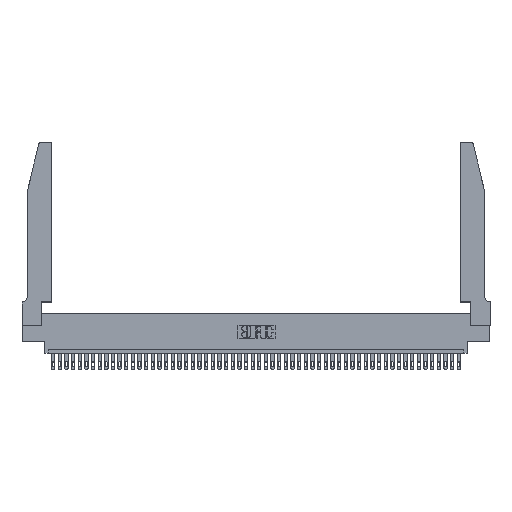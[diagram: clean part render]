
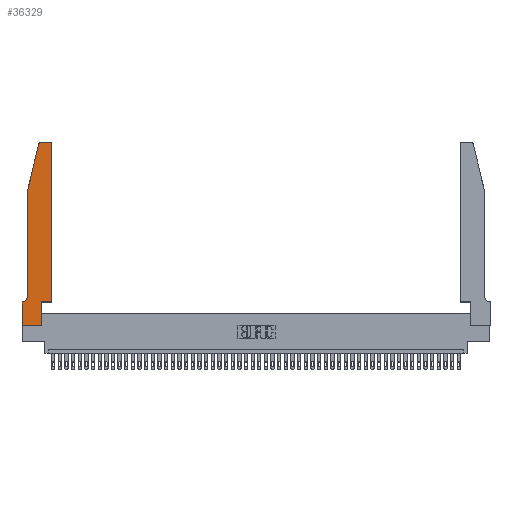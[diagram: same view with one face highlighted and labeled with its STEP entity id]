
A CAD part, top view. The second image highlights one B-rep face of the part: STEP entity #36329.
In plain terms, the highlighted planar face has unit normal (0, 0, 1).
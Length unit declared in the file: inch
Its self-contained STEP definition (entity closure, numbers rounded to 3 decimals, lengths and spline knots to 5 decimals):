
#313 = LINE ( 'NONE', #13249, #35211 ) ;
#465 = ORIENTED_EDGE ( 'NONE', *, *, #33713, .T. ) ;
#1014 = EDGE_CURVE ( 'NONE', #37259, #3808, #41794, .T. ) ;
#1759 = EDGE_CURVE ( 'NONE', #17197, #36417, #34641, .T. ) ;
#2037 = CARTESIAN_POINT ( 'NONE',  ( 0.2865, 0., 0.37 ) ) ;
#3360 = CARTESIAN_POINT ( 'NONE',  ( 0.0055, 0.42, 0.37 ) ) ;
#3808 = VERTEX_POINT ( 'NONE', #19038 ) ;
#4609 = VECTOR ( 'NONE', #18276, 39.37008 ) ;
#5124 = CARTESIAN_POINT ( 'NONE',  ( 0.2865, 0.35, 0.37 ) ) ;
#5352 = CARTESIAN_POINT ( 'NONE',  ( 0.4505, 0.35, 0.37 ) ) ;
#5495 = DIRECTION ( 'NONE',  ( 1., 0., 0. ) ) ;
#6213 = CARTESIAN_POINT ( 'NONE',  ( 0.0055, 0.35, 0.37 ) ) ;
#6795 = ORIENTED_EDGE ( 'NONE', *, *, #1014, .T. ) ;
#7836 = VECTOR ( 'NONE', #42187, 39.37008 ) ;
#8555 = VECTOR ( 'NONE', #39534, 39.37008 ) ;
#8601 = CARTESIAN_POINT ( 'NONE',  ( 0., 0., 0.37 ) ) ;
#8761 = VECTOR ( 'NONE', #44120, 39.37008 ) ;
#9191 = LINE ( 'NONE', #18901, #4609 ) ;
#10283 = DIRECTION ( 'NONE',  ( 0., 0., -1. ) ) ;
#10399 = CARTESIAN_POINT ( 'NONE',  ( 0.284, 2.72, 0.37 ) ) ;
#10502 = CARTESIAN_POINT ( 'NONE',  ( 0.4505, 0.35, 0.37 ) ) ;
#11768 = EDGE_CURVE ( 'NONE', #13589, #13318, #48666, .T. ) ;
#13249 = CARTESIAN_POINT ( 'NONE',  ( 0., 0., 0.37 ) ) ;
#13318 = VERTEX_POINT ( 'NONE', #17621 ) ;
#13589 = VERTEX_POINT ( 'NONE', #18974 ) ;
#13958 = AXIS2_PLACEMENT_3D ( 'NONE', #16506, #35367, #42558 ) ;
#14558 = DIRECTION ( 'NONE',  ( -1., 0., 0. ) ) ;
#15835 = DIRECTION ( 'NONE',  ( -1., 0., 0. ) ) ;
#16033 = ORIENTED_EDGE ( 'NONE', *, *, #34272, .T. ) ;
#16506 = CARTESIAN_POINT ( 'NONE',  ( 0.4205, 2.72, 0.37 ) ) ;
#16645 = EDGE_CURVE ( 'NONE', #3808, #44505, #39699, .T. ) ;
#17197 = VERTEX_POINT ( 'NONE', #47738 ) ;
#17353 = VECTOR ( 'NONE', #38333, 39.37008 ) ;
#17621 = CARTESIAN_POINT ( 'NONE',  ( 0.4505, 2.72, 0.37 ) ) ;
#18165 = EDGE_LOOP ( 'NONE', ( #6795, #29452, #19487, #28990, #40394, #465, #42507, #39219, #21370, #43020, #37192, #16033 ) ) ;
#18276 = DIRECTION ( 'NONE',  ( 0., -1., 0. ) ) ;
#18901 = CARTESIAN_POINT ( 'NONE',  ( 0.0755, 2., 0.37 ) ) ;
#18955 = DIRECTION ( 'NONE',  ( 0., 0., 1. ) ) ;
#18974 = CARTESIAN_POINT ( 'NONE',  ( 0.4505, 0.35, 0.37 ) ) ;
#19038 = CARTESIAN_POINT ( 'NONE',  ( 0.284, 2.75, 0.37 ) ) ;
#19401 = CIRCLE ( 'NONE', #13958, 0.03 ) ;
#19487 = ORIENTED_EDGE ( 'NONE', *, *, #44475, .T. ) ;
#20638 = VERTEX_POINT ( 'NONE', #2037 ) ;
#20830 = VERTEX_POINT ( 'NONE', #39333 ) ;
#21370 = ORIENTED_EDGE ( 'NONE', *, *, #22232, .T. ) ;
#21866 = DIRECTION ( 'NONE',  ( -1., 0., 0. ) ) ;
#22232 = EDGE_CURVE ( 'NONE', #20638, #30348, #48543, .T. ) ;
#22939 = VECTOR ( 'NONE', #21866, 39.37008 ) ;
#25024 = AXIS2_PLACEMENT_3D ( 'NONE', #3360, #10283, #14558 ) ;
#25936 = VERTEX_POINT ( 'NONE', #34580 ) ;
#28990 = ORIENTED_EDGE ( 'NONE', *, *, #44555, .T. ) ;
#29007 = AXIS2_PLACEMENT_3D ( 'NONE', #34801, #18955, #45269 ) ;
#29351 = CARTESIAN_POINT ( 'NONE',  ( 0.0755, 2., 0.37 ) ) ;
#29452 = ORIENTED_EDGE ( 'NONE', *, *, #16645, .T. ) ;
#29486 = EDGE_CURVE ( 'NONE', #37137, #20638, #313, .T. ) ;
#30118 = LINE ( 'NONE', #29351, #8761 ) ;
#30348 = VERTEX_POINT ( 'NONE', #5124 ) ;
#31714 = PLANE ( 'NONE',  #29007 ) ;
#32762 = AXIS2_PLACEMENT_3D ( 'NONE', #10399, #43868, #44190 ) ;
#33713 = EDGE_CURVE ( 'NONE', #36417, #25936, #41875, .T. ) ;
#34272 = EDGE_CURVE ( 'NONE', #13318, #37259, #19401, .T. ) ;
#34346 = DIRECTION ( 'NONE',  ( 0., -1., 0. ) ) ;
#34580 = CARTESIAN_POINT ( 'NONE',  ( 0., 0.35, 0.37 ) ) ;
#34641 = CIRCLE ( 'NONE', #25024, 0.07 ) ;
#34694 = CARTESIAN_POINT ( 'NONE',  ( 0.0755, 0.35, 0.37 ) ) ;
#34801 = CARTESIAN_POINT ( 'NONE',  ( 0., 0.35, 0.37 ) ) ;
#35211 = VECTOR ( 'NONE', #5495, 39.37008 ) ;
#35217 = FACE_OUTER_BOUND ( 'NONE', #18165, .T. ) ;
#35367 = DIRECTION ( 'NONE',  ( 0., 0., 1. ) ) ;
#36329 = ADVANCED_FACE ( 'NONE', ( #35217 ), #31714, .T. ) ;
#36417 = VERTEX_POINT ( 'NONE', #6213 ) ;
#36899 = CARTESIAN_POINT ( 'NONE',  ( 0.2605, 2.75, 0.37 ) ) ;
#37137 = VERTEX_POINT ( 'NONE', #8601 ) ;
#37192 = ORIENTED_EDGE ( 'NONE', *, *, #11768, .T. ) ;
#37259 = VERTEX_POINT ( 'NONE', #43404 ) ;
#38333 = DIRECTION ( 'NONE',  ( 1., 0., 0. ) ) ;
#38565 = EDGE_CURVE ( 'NONE', #30348, #13589, #46735, .T. ) ;
#38718 = LINE ( 'NONE', #45782, #39927 ) ;
#39219 = ORIENTED_EDGE ( 'NONE', *, *, #29486, .T. ) ;
#39333 = CARTESIAN_POINT ( 'NONE',  ( 0.0755, 2., 0.37 ) ) ;
#39534 = DIRECTION ( 'NONE',  ( 0., 1., 0. ) ) ;
#39699 = CIRCLE ( 'NONE', #32762, 0.03 ) ;
#39927 = VECTOR ( 'NONE', #34346, 39.37008 ) ;
#40394 = ORIENTED_EDGE ( 'NONE', *, *, #1759, .T. ) ;
#41794 = LINE ( 'NONE', #36899, #22939 ) ;
#41875 = LINE ( 'NONE', #34694, #45371 ) ;
#42187 = DIRECTION ( 'NONE',  ( 0., 1., 0. ) ) ;
#42507 = ORIENTED_EDGE ( 'NONE', *, *, #46724, .T. ) ;
#42558 = DIRECTION ( 'NONE',  ( 1., 0., 0. ) ) ;
#43020 = ORIENTED_EDGE ( 'NONE', *, *, #38565, .T. ) ;
#43404 = CARTESIAN_POINT ( 'NONE',  ( 0.4205, 2.75, 0.37 ) ) ;
#43868 = DIRECTION ( 'NONE',  ( 0., 0., 1. ) ) ;
#43970 = CARTESIAN_POINT ( 'NONE',  ( 0.25487, 2.72718, 0.37 ) ) ;
#44120 = DIRECTION ( 'NONE',  ( -0.239, -0.971, 0. ) ) ;
#44190 = DIRECTION ( 'NONE',  ( 1., 0., 0. ) ) ;
#44475 = EDGE_CURVE ( 'NONE', #44505, #20830, #30118, .T. ) ;
#44505 = VERTEX_POINT ( 'NONE', #43970 ) ;
#44555 = EDGE_CURVE ( 'NONE', #20830, #17197, #9191, .T. ) ;
#45269 = DIRECTION ( 'NONE',  ( 1., 0., 0. ) ) ;
#45319 = CARTESIAN_POINT ( 'NONE',  ( 0.2865, 0.35, 0.37 ) ) ;
#45371 = VECTOR ( 'NONE', #15835, 39.37008 ) ;
#45782 = CARTESIAN_POINT ( 'NONE',  ( 0., 0., 0.37 ) ) ;
#46724 = EDGE_CURVE ( 'NONE', #25936, #37137, #38718, .T. ) ;
#46735 = LINE ( 'NONE', #10502, #17353 ) ;
#47738 = CARTESIAN_POINT ( 'NONE',  ( 0.0755, 0.42, 0.37 ) ) ;
#48543 = LINE ( 'NONE', #45319, #7836 ) ;
#48666 = LINE ( 'NONE', #5352, #8555 ) ;
